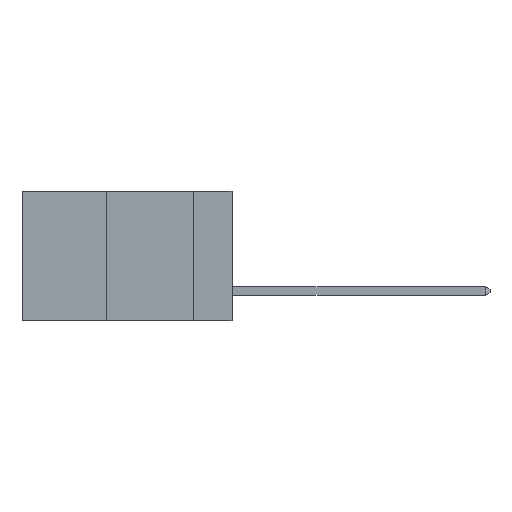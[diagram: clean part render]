
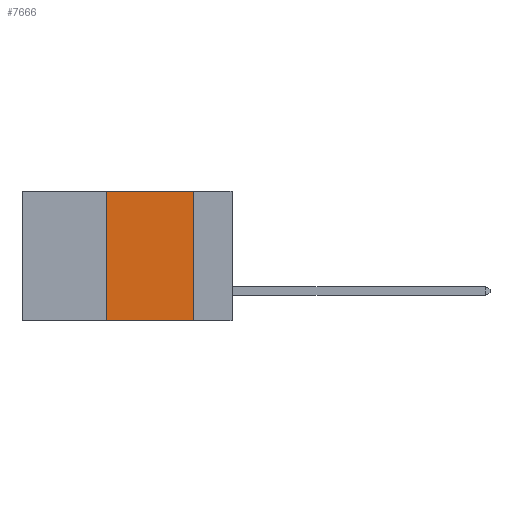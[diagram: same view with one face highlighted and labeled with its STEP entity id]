
A CAD part, left-side view. The second image highlights one B-rep face of the part: STEP entity #7666.
In plain terms, the highlighted planar face has unit normal (-1, 0, 0).
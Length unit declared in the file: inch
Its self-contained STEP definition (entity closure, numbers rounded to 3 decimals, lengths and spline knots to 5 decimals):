
#81 = CARTESIAN_POINT ( 'NONE',  ( 0., 0.6, 0. ) ) ;
#177 = LINE ( 'NONE', #81, #5723 ) ;
#195 = VERTEX_POINT ( 'NONE', #2243 ) ;
#286 = DIRECTION ( 'NONE',  ( 0., 0., -1. ) ) ;
#994 = DIRECTION ( 'NONE',  ( 0., -1., 0. ) ) ;
#1054 = VERTEX_POINT ( 'NONE', #10022 ) ;
#1733 = EDGE_CURVE ( 'NONE', #195, #5206, #7277, .T. ) ;
#2243 = CARTESIAN_POINT ( 'NONE',  ( 0., 0.11, 0. ) ) ;
#3459 = CARTESIAN_POINT ( 'NONE',  ( 0., 0.11, 0. ) ) ;
#4383 = CARTESIAN_POINT ( 'NONE',  ( 0., 0.36, -0.37 ) ) ;
#4883 = VECTOR ( 'NONE', #994, 39.37008 ) ;
#5206 = VERTEX_POINT ( 'NONE', #9423 ) ;
#5574 = FACE_OUTER_BOUND ( 'NONE', #12602, .T. ) ;
#5723 = VECTOR ( 'NONE', #8719, 39.37008 ) ;
#5799 = PLANE ( 'NONE',  #11687 ) ;
#6861 = DIRECTION ( 'NONE',  ( 1., 0., 0. ) ) ;
#7277 = LINE ( 'NONE', #3459, #9627 ) ;
#7532 = CARTESIAN_POINT ( 'NONE',  ( 0., 0.6, -0.37 ) ) ;
#7666 = ADVANCED_FACE ( 'NONE', ( #5574 ), #5799, .F. ) ;
#8719 = DIRECTION ( 'NONE',  ( 0., -1., 0. ) ) ;
#9024 = CARTESIAN_POINT ( 'NONE',  ( 0., 0.36, 0. ) ) ;
#9423 = CARTESIAN_POINT ( 'NONE',  ( 0., 0.11, -0.37 ) ) ;
#9627 = VECTOR ( 'NONE', #11553, 39.37008 ) ;
#9884 = VECTOR ( 'NONE', #12067, 39.37008 ) ;
#10022 = CARTESIAN_POINT ( 'NONE',  ( 0., 0.36, 0. ) ) ;
#10176 = VERTEX_POINT ( 'NONE', #4383 ) ;
#10446 = ORIENTED_EDGE ( 'NONE', *, *, #11183, .F. ) ;
#11183 = EDGE_CURVE ( 'NONE', #10176, #1054, #12860, .T. ) ;
#11494 = ORIENTED_EDGE ( 'NONE', *, *, #11567, .F. ) ;
#11553 = DIRECTION ( 'NONE',  ( 0., 0., -1. ) ) ;
#11567 = EDGE_CURVE ( 'NONE', #1054, #195, #177, .T. ) ;
#11606 = ORIENTED_EDGE ( 'NONE', *, *, #12782, .T. ) ;
#11687 = AXIS2_PLACEMENT_3D ( 'NONE', #11886, #6861, #286 ) ;
#11722 = ORIENTED_EDGE ( 'NONE', *, *, #1733, .F. ) ;
#11886 = CARTESIAN_POINT ( 'NONE',  ( 0., 0.6, 0. ) ) ;
#12067 = DIRECTION ( 'NONE',  ( 0., 0., 1. ) ) ;
#12602 = EDGE_LOOP ( 'NONE', ( #11722, #11494, #10446, #11606 ) ) ;
#12674 = LINE ( 'NONE', #7532, #4883 ) ;
#12782 = EDGE_CURVE ( 'NONE', #10176, #5206, #12674, .T. ) ;
#12860 = LINE ( 'NONE', #9024, #9884 ) ;
